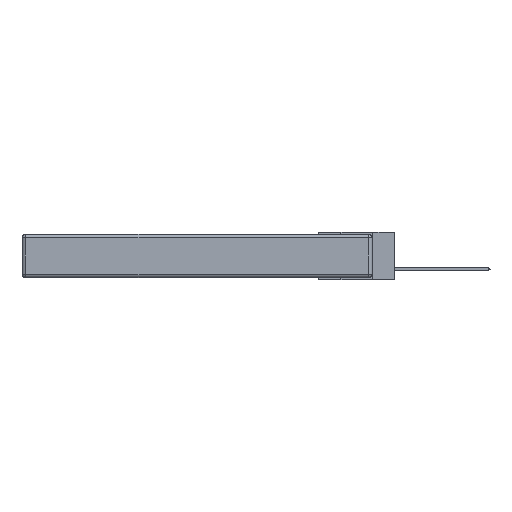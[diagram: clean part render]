
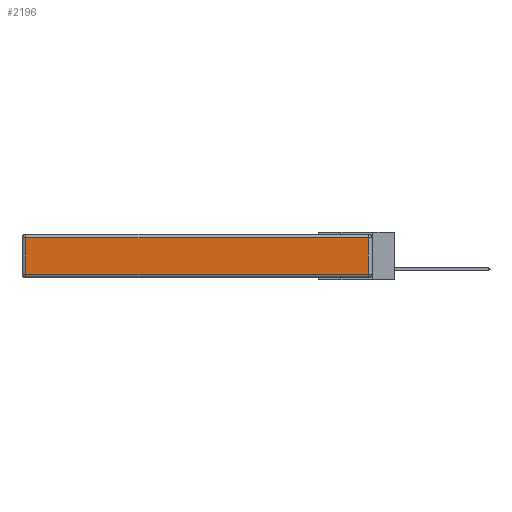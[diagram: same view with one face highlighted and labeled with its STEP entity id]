
A CAD part, left-side view. The second image highlights one B-rep face of the part: STEP entity #2196.
In plain terms, the highlighted planar face has unit normal (-1, 0, 0).
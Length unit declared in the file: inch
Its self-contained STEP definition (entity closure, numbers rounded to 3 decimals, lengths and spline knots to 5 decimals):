
#2196 = ADVANCED_FACE ( 'NONE', ( #29026 ), #31450, .T. ) ;
#2696 = CARTESIAN_POINT ( 'NONE',  ( 0., 2.72, -0.03 ) ) ;
#2859 = CARTESIAN_POINT ( 'NONE',  ( 0., 0., -0.343 ) ) ;
#3014 = ORIENTED_EDGE ( 'NONE', *, *, #33030, .T. ) ;
#4162 = CARTESIAN_POINT ( 'NONE',  ( 0., 0.03, -0.03 ) ) ;
#4700 = DIRECTION ( 'NONE',  ( 0., 1., 0. ) ) ;
#4915 = CARTESIAN_POINT ( 'NONE',  ( 0., 2.75, -0.03 ) ) ;
#5189 = EDGE_CURVE ( 'NONE', #10578, #31588, #9331, .T. ) ;
#6208 = DIRECTION ( 'NONE',  ( 0., -1., 0. ) ) ;
#6604 = VECTOR ( 'NONE', #23920, 39.37008 ) ;
#8232 = LINE ( 'NONE', #31433, #18287 ) ;
#9331 = LINE ( 'NONE', #4915, #27083 ) ;
#9455 = ORIENTED_EDGE ( 'NONE', *, *, #23602, .T. ) ;
#10578 = VERTEX_POINT ( 'NONE', #4162 ) ;
#14976 = CARTESIAN_POINT ( 'NONE',  ( 0., 0.03, -0.313 ) ) ;
#15428 = LINE ( 'NONE', #18857, #6604 ) ;
#15434 = EDGE_LOOP ( 'NONE', ( #3014, #23342, #18347, #9455 ) ) ;
#15513 = DIRECTION ( 'NONE',  ( 0., 0., 1. ) ) ;
#16687 = AXIS2_PLACEMENT_3D ( 'NONE', #2859, #23329, #28867 ) ;
#18287 = VECTOR ( 'NONE', #15513, 39.37008 ) ;
#18347 = ORIENTED_EDGE ( 'NONE', *, *, #5189, .T. ) ;
#18857 = CARTESIAN_POINT ( 'NONE',  ( 0., 2.72, -0.343 ) ) ;
#19079 = EDGE_CURVE ( 'NONE', #27292, #10578, #8232, .T. ) ;
#23329 = DIRECTION ( 'NONE',  ( -1., 0., 0. ) ) ;
#23342 = ORIENTED_EDGE ( 'NONE', *, *, #19079, .T. ) ;
#23602 = EDGE_CURVE ( 'NONE', #31588, #24170, #15428, .T. ) ;
#23892 = CARTESIAN_POINT ( 'NONE',  ( 0., 0., -0.313 ) ) ;
#23920 = DIRECTION ( 'NONE',  ( 0., 0., -1. ) ) ;
#24170 = VERTEX_POINT ( 'NONE', #26112 ) ;
#26112 = CARTESIAN_POINT ( 'NONE',  ( 0., 2.72, -0.313 ) ) ;
#27024 = LINE ( 'NONE', #23892, #31089 ) ;
#27083 = VECTOR ( 'NONE', #4700, 39.37008 ) ;
#27292 = VERTEX_POINT ( 'NONE', #14976 ) ;
#28867 = DIRECTION ( 'NONE',  ( 0., 0., 1. ) ) ;
#29026 = FACE_OUTER_BOUND ( 'NONE', #15434, .T. ) ;
#31089 = VECTOR ( 'NONE', #6208, 39.37008 ) ;
#31433 = CARTESIAN_POINT ( 'NONE',  ( 0., 0.03, -0.343 ) ) ;
#31450 = PLANE ( 'NONE',  #16687 ) ;
#31588 = VERTEX_POINT ( 'NONE', #2696 ) ;
#33030 = EDGE_CURVE ( 'NONE', #24170, #27292, #27024, .T. ) ;
